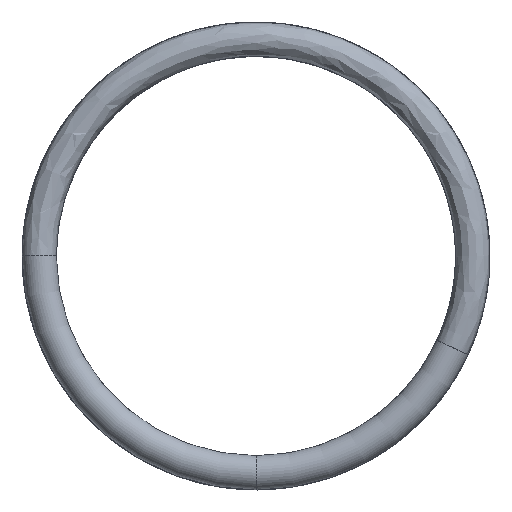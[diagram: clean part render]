
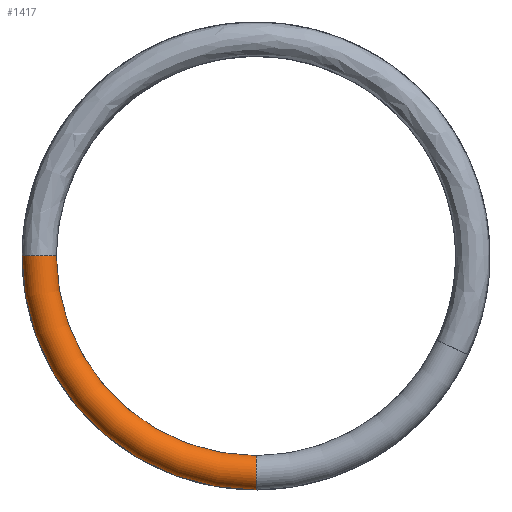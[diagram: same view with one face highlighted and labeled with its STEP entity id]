
A CAD part, front view. The second image highlights one B-rep face of the part: STEP entity #1417.
In plain terms, the highlighted toroidal (fillet/blend) face has major radius 2.407 mm and minor radius 0.191 mm.
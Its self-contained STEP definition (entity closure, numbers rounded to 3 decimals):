
#295 = ORIENTED_EDGE ( 'NONE', *, *, #4297, .T. ) ;
#351 = CARTESIAN_POINT ( 'NONE',  ( -2.597, 0.191, 0. ) ) ;
#661 = TOROIDAL_SURFACE ( 'NONE', #4901, 2.407, 0.191 ) ;
#727 = CARTESIAN_POINT ( 'NONE',  ( 0., 0.191, -2.407 ) ) ;
#777 = DIRECTION ( 'NONE',  ( 0., -1., 0. ) ) ;
#841 = CARTESIAN_POINT ( 'NONE',  ( 0., 0.191, -2.597 ) ) ;
#917 = CARTESIAN_POINT ( 'NONE',  ( 0., 0.191, 0. ) ) ;
#947 = CIRCLE ( 'NONE', #4310, 2.597 ) ;
#1099 = CARTESIAN_POINT ( 'NONE',  ( -2.216, 0.191, 0. ) ) ;
#1118 = DIRECTION ( 'NONE',  ( 0., 0., 1. ) ) ;
#1174 = DIRECTION ( 'NONE',  ( 0., 0., -1. ) ) ;
#1353 = ORIENTED_EDGE ( 'NONE', *, *, #1787, .F. ) ;
#1417 = ADVANCED_FACE ( 'NONE', ( #1677 ), #661, .T. ) ;
#1506 = CARTESIAN_POINT ( 'NONE',  ( -2.237, 0.091, 0. ) ) ;
#1677 = FACE_OUTER_BOUND ( 'NONE', #2291, .T. ) ;
#1787 = EDGE_CURVE ( 'NONE', #2310, #3275, #1813, .T. ) ;
#1813 = CIRCLE ( 'NONE', #4790, 2.216 ) ;
#1899 = CARTESIAN_POINT ( 'NONE',  ( -2.357, 0., 0. ) ) ;
#2090 = CIRCLE ( 'NONE', #4439, 0.191 ) ;
#2139 = ORIENTED_EDGE ( 'NONE', *, *, #3708, .T. ) ;
#2275 = CARTESIAN_POINT ( 'NONE',  ( -2.506, 0.021, 0. ) ) ;
#2291 = EDGE_LOOP ( 'NONE', ( #3401, #295, #2139, #1353 ) ) ;
#2310 = VERTEX_POINT ( 'NONE', #3481 ) ;
#2353 = DIRECTION ( 'NONE',  ( 0., -1., 0. ) ) ;
#2376 = VERTEX_POINT ( 'NONE', #3122 ) ;
#2513 = VERTEX_POINT ( 'NONE', #841 ) ;
#2655 = CARTESIAN_POINT ( 'NONE',  ( -2.597, 0.141, 0. ) ) ;
#2925 = B_SPLINE_CURVE_WITH_KNOTS ( 'NONE', 3,
 ( #1099, #4900, #1506, #4143, #1899, #4529, #2275, #4920, #2655, #351 ),
 .UNSPECIFIED., .F., .F.,
 ( 4, 2, 2, 2, 4 ),
 ( 0., 0.25, 0.5, 0.75, 1. ),
 .UNSPECIFIED. ) ;
#3060 = CARTESIAN_POINT ( 'NONE',  ( 0., 0.191, 0. ) ) ;
#3122 = CARTESIAN_POINT ( 'NONE',  ( -2.597, 0.191, 0. ) ) ;
#3275 = VERTEX_POINT ( 'NONE', #3462 ) ;
#3382 = DIRECTION ( 'NONE',  ( -1., 0., 0. ) ) ;
#3401 = ORIENTED_EDGE ( 'NONE', *, *, #3807, .T. ) ;
#3427 = DIRECTION ( 'NONE',  ( 0., 0., -1. ) ) ;
#3436 = DIRECTION ( 'NONE',  ( 0., -1., 0. ) ) ;
#3462 = CARTESIAN_POINT ( 'NONE',  ( 0., 0.191, -2.216 ) ) ;
#3481 = CARTESIAN_POINT ( 'NONE',  ( -2.216, 0.191, 0. ) ) ;
#3708 = EDGE_CURVE ( 'NONE', #2513, #3275, #2090, .T. ) ;
#3807 = EDGE_CURVE ( 'NONE', #2310, #2376, #2925, .T. ) ;
#4143 = CARTESIAN_POINT ( 'NONE',  ( -2.307, 0.021, 0. ) ) ;
#4241 = DIRECTION ( 'NONE',  ( 0., 0., -1. ) ) ;
#4297 = EDGE_CURVE ( 'NONE', #2376, #2513, #947, .T. ) ;
#4310 = AXIS2_PLACEMENT_3D ( 'NONE', #3060, #777, #3427 ) ;
#4439 = AXIS2_PLACEMENT_3D ( 'NONE', #727, #3382, #1118 ) ;
#4529 = CARTESIAN_POINT ( 'NONE',  ( -2.457, 0., 0. ) ) ;
#4631 = CARTESIAN_POINT ( 'NONE',  ( 0., 0.191, 0. ) ) ;
#4790 = AXIS2_PLACEMENT_3D ( 'NONE', #4631, #3436, #1174 ) ;
#4900 = CARTESIAN_POINT ( 'NONE',  ( -2.216, 0.141, 0. ) ) ;
#4901 = AXIS2_PLACEMENT_3D ( 'NONE', #917, #2353, #4241 ) ;
#4920 = CARTESIAN_POINT ( 'NONE',  ( -2.577, 0.091, 0. ) ) ;
